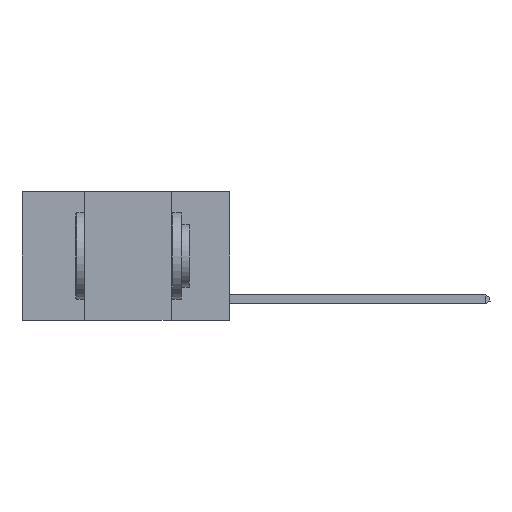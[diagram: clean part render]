
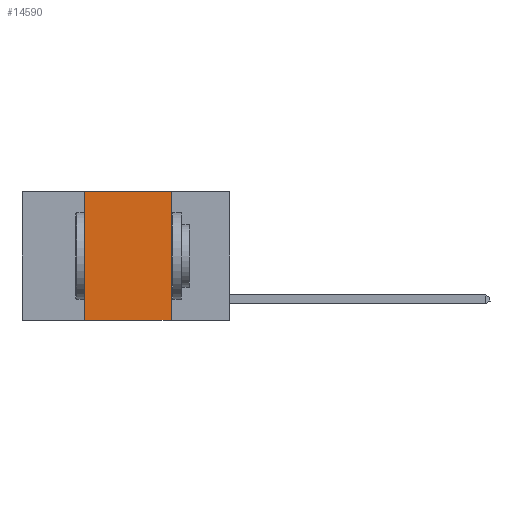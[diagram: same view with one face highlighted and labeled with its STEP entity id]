
A CAD part, left-side view. The second image highlights one B-rep face of the part: STEP entity #14590.
In plain terms, the highlighted planar face has unit normal (-1, 0, 0).
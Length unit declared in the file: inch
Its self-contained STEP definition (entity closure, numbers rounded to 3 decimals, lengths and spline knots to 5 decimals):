
#271 = CARTESIAN_POINT ( 'NONE',  ( 0., 0.17, 0. ) ) ;
#674 = DIRECTION ( 'NONE',  ( 1., 0., 0. ) ) ;
#1095 = EDGE_CURVE ( 'NONE', #12868, #27144, #3553, .T. ) ;
#1336 = VECTOR ( 'NONE', #8298, 39.37008 ) ;
#1593 = DIRECTION ( 'NONE',  ( 0., -1., 0. ) ) ;
#1776 = CARTESIAN_POINT ( 'NONE',  ( 0., 0.42, 0. ) ) ;
#1966 = CARTESIAN_POINT ( 'NONE',  ( 0., 0.6, -0.37 ) ) ;
#2451 = EDGE_LOOP ( 'NONE', ( #8639, #20847, #9184, #19799 ) ) ;
#2927 = CARTESIAN_POINT ( 'NONE',  ( 0., 0.42, 0. ) ) ;
#3553 = LINE ( 'NONE', #1966, #19661 ) ;
#4673 = DIRECTION ( 'NONE',  ( 0., 0., -1. ) ) ;
#4780 = CARTESIAN_POINT ( 'NONE',  ( 0., 0.17, 0. ) ) ;
#6107 = CARTESIAN_POINT ( 'NONE',  ( 0., 0.6, 0. ) ) ;
#6255 = FACE_OUTER_BOUND ( 'NONE', #2451, .T. ) ;
#6843 = EDGE_CURVE ( 'NONE', #12868, #17589, #7894, .T. ) ;
#7894 = LINE ( 'NONE', #1776, #1336 ) ;
#8285 = EDGE_CURVE ( 'NONE', #18809, #27144, #8811, .T. ) ;
#8298 = DIRECTION ( 'NONE',  ( 0., 0., 1. ) ) ;
#8639 = ORIENTED_EDGE ( 'NONE', *, *, #8285, .F. ) ;
#8811 = LINE ( 'NONE', #271, #13966 ) ;
#9184 = ORIENTED_EDGE ( 'NONE', *, *, #6843, .F. ) ;
#11557 = LINE ( 'NONE', #6107, #24341 ) ;
#11566 = CARTESIAN_POINT ( 'NONE',  ( 0., 0.6, 0. ) ) ;
#12868 = VERTEX_POINT ( 'NONE', #23725 ) ;
#13966 = VECTOR ( 'NONE', #4673, 39.37008 ) ;
#14590 = ADVANCED_FACE ( 'NONE', ( #6255 ), #26899, .F. ) ;
#15983 = DIRECTION ( 'NONE',  ( 0., 0., -1. ) ) ;
#16934 = CARTESIAN_POINT ( 'NONE',  ( 0., 0.17, -0.37 ) ) ;
#17589 = VERTEX_POINT ( 'NONE', #2927 ) ;
#18809 = VERTEX_POINT ( 'NONE', #4780 ) ;
#19661 = VECTOR ( 'NONE', #1593, 39.37008 ) ;
#19799 = ORIENTED_EDGE ( 'NONE', *, *, #1095, .T. ) ;
#20847 = ORIENTED_EDGE ( 'NONE', *, *, #23057, .F. ) ;
#23057 = EDGE_CURVE ( 'NONE', #17589, #18809, #11557, .T. ) ;
#23515 = AXIS2_PLACEMENT_3D ( 'NONE', #11566, #674, #15983 ) ;
#23725 = CARTESIAN_POINT ( 'NONE',  ( 0., 0.42, -0.37 ) ) ;
#24341 = VECTOR ( 'NONE', #27997, 39.37008 ) ;
#26899 = PLANE ( 'NONE',  #23515 ) ;
#27144 = VERTEX_POINT ( 'NONE', #16934 ) ;
#27997 = DIRECTION ( 'NONE',  ( 0., -1., 0. ) ) ;
